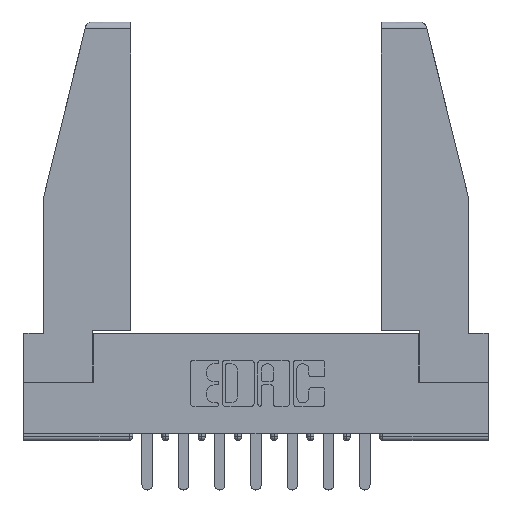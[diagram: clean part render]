
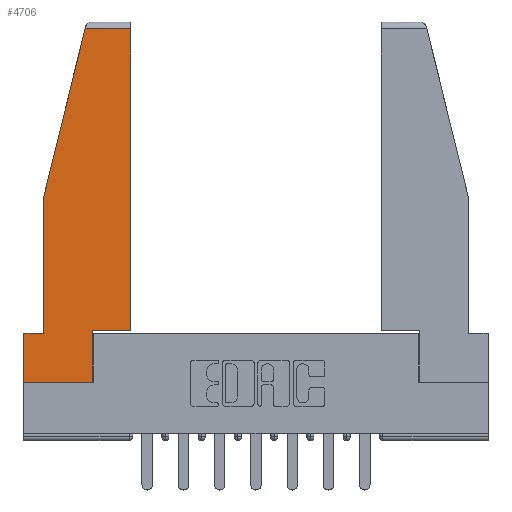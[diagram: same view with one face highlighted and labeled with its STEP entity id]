
A CAD part, top view. The second image highlights one B-rep face of the part: STEP entity #4706.
In plain terms, the highlighted planar face has unit normal (0, 0, 1).
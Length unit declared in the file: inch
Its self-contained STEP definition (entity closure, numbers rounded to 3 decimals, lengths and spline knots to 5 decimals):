
#61 = EDGE_CURVE ( 'NONE', #2327, #5990, #6346, .T. ) ;
#124 = EDGE_CURVE ( 'NONE', #3168, #2585, #10512, .T. ) ;
#190 = DIRECTION ( 'NONE',  ( 0., -1., 0. ) ) ;
#733 = CARTESIAN_POINT ( 'NONE',  ( 0., 0.21, 0. ) ) ;
#865 = ORIENTED_EDGE ( 'NONE', *, *, #2340, .T. ) ;
#1027 = CARTESIAN_POINT ( 'NONE',  ( 0.086, 0.21, 0. ) ) ;
#1126 = CARTESIAN_POINT ( 'NONE',  ( 0.086, 0.8, 0. ) ) ;
#1409 = VECTOR ( 'NONE', #11484, 39.37008 ) ;
#1717 = CARTESIAN_POINT ( 'NONE',  ( 0.297, 0.223, 0. ) ) ;
#2152 = CARTESIAN_POINT ( 'NONE',  ( 0.271, 1.55, 0. ) ) ;
#2162 = ORIENTED_EDGE ( 'NONE', *, *, #11863, .T. ) ;
#2204 = DIRECTION ( 'NONE',  ( -0.239, -0.971, 0. ) ) ;
#2327 = VERTEX_POINT ( 'NONE', #8974 ) ;
#2340 = EDGE_CURVE ( 'NONE', #10598, #3168, #5707, .T. ) ;
#2538 = ORIENTED_EDGE ( 'NONE', *, *, #8024, .T. ) ;
#2585 = VERTEX_POINT ( 'NONE', #733 ) ;
#2831 = CARTESIAN_POINT ( 'NONE',  ( 0., 0.21, 0. ) ) ;
#3168 = VERTEX_POINT ( 'NONE', #1027 ) ;
#3799 = CARTESIAN_POINT ( 'NONE',  ( 0., 1.52, 0. ) ) ;
#4263 = VERTEX_POINT ( 'NONE', #12501 ) ;
#4394 = DIRECTION ( 'NONE',  ( 0., 1., 0. ) ) ;
#4424 = CARTESIAN_POINT ( 'NONE',  ( 0., 0.21, 0. ) ) ;
#4706 = ADVANCED_FACE ( 'NONE', ( #12177 ), #6809, .T. ) ;
#4755 = CARTESIAN_POINT ( 'NONE',  ( 0.2636, 1.52, 0. ) ) ;
#4987 = DIRECTION ( 'NONE',  ( -1., 0., 0. ) ) ;
#4997 = CARTESIAN_POINT ( 'NONE',  ( 0., 0., 0. ) ) ;
#5084 = VECTOR ( 'NONE', #4394, 39.37008 ) ;
#5311 = EDGE_LOOP ( 'NONE', ( #11774, #5911, #2162, #865, #9571, #8555, #5807, #2538, #10620 ) ) ;
#5508 = DIRECTION ( 'NONE',  ( 1., 0., 0. ) ) ;
#5577 = VERTEX_POINT ( 'NONE', #13595 ) ;
#5595 = AXIS2_PLACEMENT_3D ( 'NONE', #13328, #11052, #7920 ) ;
#5701 = CARTESIAN_POINT ( 'NONE',  ( 0.086, 0.8, 0. ) ) ;
#5707 = LINE ( 'NONE', #1126, #8311 ) ;
#5807 = ORIENTED_EDGE ( 'NONE', *, *, #14073, .T. ) ;
#5911 = ORIENTED_EDGE ( 'NONE', *, *, #61, .T. ) ;
#5990 = VERTEX_POINT ( 'NONE', #4755 ) ;
#6124 = VERTEX_POINT ( 'NONE', #4997 ) ;
#6346 = LINE ( 'NONE', #3799, #1409 ) ;
#6809 = PLANE ( 'NONE',  #5595 ) ;
#7073 = EDGE_CURVE ( 'NONE', #7469, #5577, #11833, .T. ) ;
#7469 = VERTEX_POINT ( 'NONE', #1717 ) ;
#7555 = VECTOR ( 'NONE', #4987, 39.37008 ) ;
#7667 = CARTESIAN_POINT ( 'NONE',  ( 0.297, 0.223, 0. ) ) ;
#7687 = LINE ( 'NONE', #13843, #12003 ) ;
#7920 = DIRECTION ( 'NONE',  ( 1., 0., 0. ) ) ;
#8024 = EDGE_CURVE ( 'NONE', #4263, #7469, #10106, .T. ) ;
#8267 = DIRECTION ( 'NONE',  ( 0., 1., 0. ) ) ;
#8311 = VECTOR ( 'NONE', #190, 39.37008 ) ;
#8555 = ORIENTED_EDGE ( 'NONE', *, *, #12989, .T. ) ;
#8683 = VECTOR ( 'NONE', #13208, 39.37008 ) ;
#8974 = CARTESIAN_POINT ( 'NONE',  ( 0.461, 1.52, 0. ) ) ;
#9145 = LINE ( 'NONE', #2152, #12378 ) ;
#9571 = ORIENTED_EDGE ( 'NONE', *, *, #124, .T. ) ;
#10106 = LINE ( 'NONE', #12298, #5084 ) ;
#10262 = LINE ( 'NONE', #4424, #8683 ) ;
#10512 = LINE ( 'NONE', #2831, #7555 ) ;
#10598 = VERTEX_POINT ( 'NONE', #5701 ) ;
#10620 = ORIENTED_EDGE ( 'NONE', *, *, #7073, .T. ) ;
#10645 = VECTOR ( 'NONE', #5508, 39.37008 ) ;
#11052 = DIRECTION ( 'NONE',  ( 0., 0., 1. ) ) ;
#11484 = DIRECTION ( 'NONE',  ( -1., 0., 0. ) ) ;
#11774 = ORIENTED_EDGE ( 'NONE', *, *, #12810, .T. ) ;
#11833 = LINE ( 'NONE', #7667, #10645 ) ;
#11863 = EDGE_CURVE ( 'NONE', #5990, #10598, #9145, .T. ) ;
#12003 = VECTOR ( 'NONE', #8267, 39.37008 ) ;
#12046 = DIRECTION ( 'NONE',  ( 1., 0., 0. ) ) ;
#12177 = FACE_OUTER_BOUND ( 'NONE', #5311, .T. ) ;
#12228 = VECTOR ( 'NONE', #12046, 39.37008 ) ;
#12298 = CARTESIAN_POINT ( 'NONE',  ( 0.297, 0., 0. ) ) ;
#12378 = VECTOR ( 'NONE', #2204, 39.37008 ) ;
#12501 = CARTESIAN_POINT ( 'NONE',  ( 0.297, 0., 0. ) ) ;
#12810 = EDGE_CURVE ( 'NONE', #5577, #2327, #7687, .T. ) ;
#12989 = EDGE_CURVE ( 'NONE', #2585, #6124, #10262, .T. ) ;
#13044 = LINE ( 'NONE', #14029, #12228 ) ;
#13208 = DIRECTION ( 'NONE',  ( 0., -1., 0. ) ) ;
#13328 = CARTESIAN_POINT ( 'NONE',  ( 0., 0., 0. ) ) ;
#13595 = CARTESIAN_POINT ( 'NONE',  ( 0.461, 0.223, 0. ) ) ;
#13843 = CARTESIAN_POINT ( 'NONE',  ( 0.461, 0.223, 0. ) ) ;
#14029 = CARTESIAN_POINT ( 'NONE',  ( 0., 0., 0. ) ) ;
#14073 = EDGE_CURVE ( 'NONE', #6124, #4263, #13044, .T. ) ;
